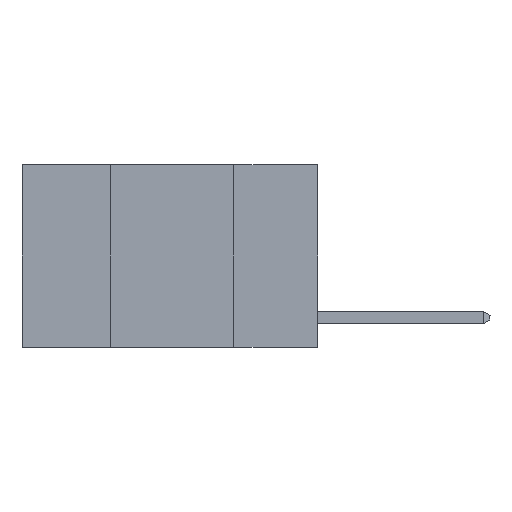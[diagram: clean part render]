
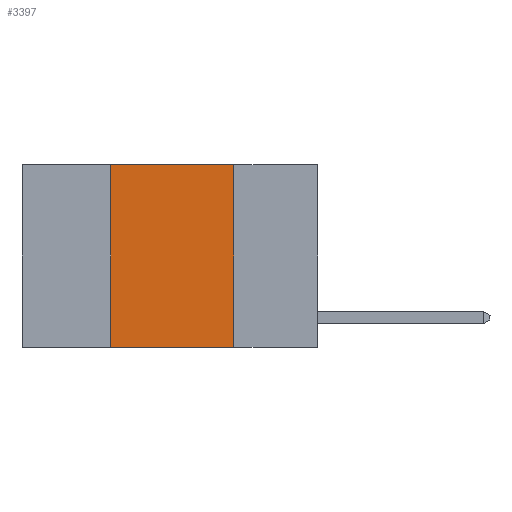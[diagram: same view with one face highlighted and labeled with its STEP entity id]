
A CAD part, left-side view. The second image highlights one B-rep face of the part: STEP entity #3397.
In plain terms, the highlighted planar face has unit normal (-1, 0, 0).
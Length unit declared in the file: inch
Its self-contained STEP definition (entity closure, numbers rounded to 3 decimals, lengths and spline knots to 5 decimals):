
#353 = CARTESIAN_POINT ( 'NONE',  ( 0., 0.42, -0.37 ) ) ;
#471 = VECTOR ( 'NONE', #9170, 39.37008 ) ;
#916 = ORIENTED_EDGE ( 'NONE', *, *, #17183, .T. ) ;
#1264 = CARTESIAN_POINT ( 'NONE',  ( 0., 0.17, -0.37 ) ) ;
#1449 = AXIS2_PLACEMENT_3D ( 'NONE', #12516, #14027, #20126 ) ;
#1794 = EDGE_CURVE ( 'NONE', #11523, #10794, #13916, .T. ) ;
#2786 = VECTOR ( 'NONE', #10802, 39.37008 ) ;
#3397 = ADVANCED_FACE ( 'NONE', ( #7821 ), #12311, .F. ) ;
#3898 = VERTEX_POINT ( 'NONE', #1264 ) ;
#4761 = EDGE_CURVE ( 'NONE', #10794, #15631, #19849, .T. ) ;
#5718 = LINE ( 'NONE', #18716, #471 ) ;
#7821 = FACE_OUTER_BOUND ( 'NONE', #15389, .T. ) ;
#8012 = LINE ( 'NONE', #9249, #18511 ) ;
#8741 = ORIENTED_EDGE ( 'NONE', *, *, #15436, .F. ) ;
#9170 = DIRECTION ( 'NONE',  ( 0., 0., -1. ) ) ;
#9249 = CARTESIAN_POINT ( 'NONE',  ( 0., 0.6, -0.37 ) ) ;
#10794 = VERTEX_POINT ( 'NONE', #15926 ) ;
#10802 = DIRECTION ( 'NONE',  ( 0., -1., 0. ) ) ;
#10888 = DIRECTION ( 'NONE',  ( 0., -1., 0. ) ) ;
#11523 = VERTEX_POINT ( 'NONE', #353 ) ;
#11525 = ORIENTED_EDGE ( 'NONE', *, *, #1794, .F. ) ;
#12311 = PLANE ( 'NONE',  #1449 ) ;
#12516 = CARTESIAN_POINT ( 'NONE',  ( 0., 0.6, 0. ) ) ;
#12595 = CARTESIAN_POINT ( 'NONE',  ( 0., 0.42, 0. ) ) ;
#13916 = LINE ( 'NONE', #12595, #19822 ) ;
#14027 = DIRECTION ( 'NONE',  ( 1., 0., 0. ) ) ;
#15389 = EDGE_LOOP ( 'NONE', ( #8741, #20077, #11525, #916 ) ) ;
#15436 = EDGE_CURVE ( 'NONE', #15631, #3898, #5718, .T. ) ;
#15631 = VERTEX_POINT ( 'NONE', #19025 ) ;
#15926 = CARTESIAN_POINT ( 'NONE',  ( 0., 0.42, 0. ) ) ;
#16826 = DIRECTION ( 'NONE',  ( 0., 0., 1. ) ) ;
#17183 = EDGE_CURVE ( 'NONE', #11523, #3898, #8012, .T. ) ;
#18402 = CARTESIAN_POINT ( 'NONE',  ( 0., 0.6, 0. ) ) ;
#18511 = VECTOR ( 'NONE', #10888, 39.37008 ) ;
#18716 = CARTESIAN_POINT ( 'NONE',  ( 0., 0.17, 0. ) ) ;
#19025 = CARTESIAN_POINT ( 'NONE',  ( 0., 0.17, 0. ) ) ;
#19822 = VECTOR ( 'NONE', #16826, 39.37008 ) ;
#19849 = LINE ( 'NONE', #18402, #2786 ) ;
#20077 = ORIENTED_EDGE ( 'NONE', *, *, #4761, .F. ) ;
#20126 = DIRECTION ( 'NONE',  ( 0., 0., -1. ) ) ;
